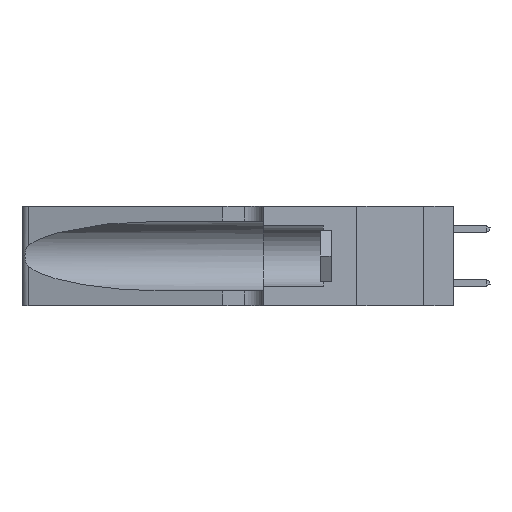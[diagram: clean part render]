
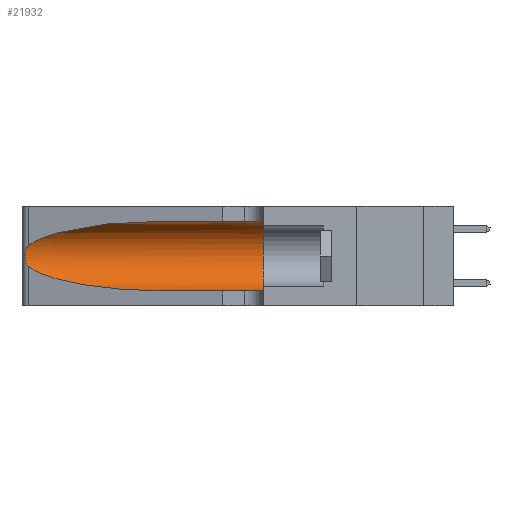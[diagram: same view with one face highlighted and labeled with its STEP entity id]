
A CAD part, left-side view. The second image highlights one B-rep face of the part: STEP entity #21932.
In plain terms, the highlighted cylindrical face has radius 3.308 mm (diameter 6.617 mm), a partial arc.
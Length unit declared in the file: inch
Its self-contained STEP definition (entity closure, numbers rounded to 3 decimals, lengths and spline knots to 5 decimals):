
#1064 = CARTESIAN_POINT ( 'NONE',  ( 0.25487, 1.22718, 0.22369 ) ) ;
#2345 = CARTESIAN_POINT ( 'NONE',  ( 0.25487, 1.22718, 0.22369 ) ) ;
#2739 = EDGE_CURVE ( 'NONE', #7046, #26798, #13587, .T. ) ;
#2786 = DIRECTION ( 'NONE',  ( 0., 0., -1. ) ) ;
#2940 = EDGE_CURVE ( 'NONE', #19266, #15660, #3195, .T. ) ;
#3195 = CIRCLE ( 'NONE', #27784, 0.13025 ) ;
#3874 = CARTESIAN_POINT ( 'NONE',  ( 0.25487, 1.22718, 0.22369 ) ) ;
#4031 = EDGE_CURVE ( 'NONE', #26867, #19266, #11959, .T. ) ;
#4232 = CYLINDRICAL_SURFACE ( 'NONE', #11273, 0.13025 ) ;
#5357 = CARTESIAN_POINT ( 'NONE',  ( 0.1305, 0.35, 0.31525 ) ) ;
#5538 = CARTESIAN_POINT ( 'NONE',  ( 0.26075, 1.23896, 0.178 ) ) ;
#5581 = VERTEX_POINT ( 'NONE', #11405 ) ;
#5630 = CARTESIAN_POINT ( 'NONE',  ( 0.26075, 1.23896, 0.19203 ) ) ;
#6467 = ORIENTED_EDGE ( 'NONE', *, *, #9641, .T. ) ;
#7046 = VERTEX_POINT ( 'NONE', #3874 ) ;
#7950 = CARTESIAN_POINT ( 'NONE',  ( 0.25854, 1.2359, 0.20912 ) ) ;
#8447 = CARTESIAN_POINT ( 'NONE',  ( 0.1305, 1.61858, 0.31525 ) ) ;
#8806 = EDGE_LOOP ( 'NONE', ( #25374, #16223, #6467, #10696, #26474, #26858 ) ) ;
#8916 = CARTESIAN_POINT ( 'NONE',  ( 0.25487, 1.22718, 0.14631 ) ) ;
#9152 = CARTESIAN_POINT ( 'NONE',  ( 0.1305, 0.35, 0.185 ) ) ;
#9641 = EDGE_CURVE ( 'NONE', #26798, #5581, #20882, .T. ) ;
#9998 = CARTESIAN_POINT ( 'NONE',  ( 0.25555, 1.22993, 0.14849 ) ) ;
#10171 = CARTESIAN_POINT ( 'NONE',  ( 0.25856, 1.23593, 0.16098 ) ) ;
#10696 = ORIENTED_EDGE ( 'NONE', *, *, #25628, .T. ) ;
#11273 = AXIS2_PLACEMENT_3D ( 'NONE', #22894, #16271, #2786 ) ;
#11405 = CARTESIAN_POINT ( 'NONE',  ( 0.1305, 0.72297, 0.05475 ) ) ;
#11941 = DIRECTION ( 'NONE',  ( 0., 0., 1. ) ) ;
#11959 = LINE ( 'NONE', #8447, #12990 ) ;
#12356 = LINE ( 'NONE', #23040, #23479 ) ;
#12990 = VECTOR ( 'NONE', #28362, 39.37008 ) ;
#13587 = B_SPLINE_CURVE_WITH_KNOTS ( 'NONE', 3,
 ( #1064, #21145, #18817, #21245, #7950, #23492, #5630, #5538, #25522, #10171, #21051, #23292, #9998, #16866 ),
 .UNSPECIFIED., .F., .F.,
 ( 4, 2, 2, 2, 2, 2, 4 ),
 ( 0., 0.00027, 0.00053, 0.00107, 0.0016, 0.00187, 0.00214 ),
 .UNSPECIFIED. ) ;
#15028 = CARTESIAN_POINT ( 'NONE',  ( 0.2373, 1.15595, 0.08982 ) ) ;
#15220 = CARTESIAN_POINT ( 'NONE',  ( 0.18966, 0.96281, 0.05475 ) ) ;
#15327 = CARTESIAN_POINT ( 'NONE',  ( 0.1305, 0.72297, 0.05475 ) ) ;
#15660 = VERTEX_POINT ( 'NONE', #19179 ) ;
#15718 = CARTESIAN_POINT ( 'NONE',  ( 0.2373, 1.15595, 0.28018 ) ) ;
#16223 = ORIENTED_EDGE ( 'NONE', *, *, #2739, .T. ) ;
#16271 = DIRECTION ( 'NONE',  ( 0., -1., 0. ) ) ;
#16866 = CARTESIAN_POINT ( 'NONE',  ( 0.25487, 1.22718, 0.14631 ) ) ;
#17584 = CARTESIAN_POINT ( 'NONE',  ( 0.1305, 0.72297, 0.31525 ) ) ;
#18536 = EDGE_CURVE ( 'NONE', #26867, #7046, #23041, .T. ) ;
#18817 = CARTESIAN_POINT ( 'NONE',  ( 0.25639, 1.23184, 0.21858 ) ) ;
#19179 = CARTESIAN_POINT ( 'NONE',  ( 0.1305, 0.35, 0.05475 ) ) ;
#19266 = VERTEX_POINT ( 'NONE', #5357 ) ;
#20882 =( BOUNDED_CURVE ( )  B_SPLINE_CURVE ( 3, ( #24077, #15028, #15220, #15327 ),
 .UNSPECIFIED., .F., .F. ) 
 B_SPLINE_CURVE_WITH_KNOTS ( ( 4, 4 ),
 ( 3.44316, 4.71239 ),
 .UNSPECIFIED. ) 
 CURVE ( )  GEOMETRIC_REPRESENTATION_ITEM ( )  RATIONAL_B_SPLINE_CURVE ( ( 1., 0.87, 0.87, 1. ) ) 
 REPRESENTATION_ITEM ( '' )  );
#21051 = CARTESIAN_POINT ( 'NONE',  ( 0.25789, 1.23486, 0.15765 ) ) ;
#21145 = CARTESIAN_POINT ( 'NONE',  ( 0.25555, 1.22994, 0.2215 ) ) ;
#21245 = CARTESIAN_POINT ( 'NONE',  ( 0.25787, 1.23484, 0.2124 ) ) ;
#21932 = ADVANCED_FACE ( 'NONE', ( #27868 ), #4232, .F. ) ;
#22651 = DIRECTION ( 'NONE',  ( 0., -1., 0. ) ) ;
#22728 = DIRECTION ( 'NONE',  ( 0., 1., 0. ) ) ;
#22894 = CARTESIAN_POINT ( 'NONE',  ( 0.1305, 1.61858, 0.185 ) ) ;
#23040 = CARTESIAN_POINT ( 'NONE',  ( 0.1305, 1.61858, 0.05475 ) ) ;
#23041 =( BOUNDED_CURVE ( )  B_SPLINE_CURVE ( 3, ( #17584, #28489, #15718, #2345 ),
 .UNSPECIFIED., .F., .F. ) 
 B_SPLINE_CURVE_WITH_KNOTS ( ( 4, 4 ),
 ( 1.5708, 2.84003 ),
 .UNSPECIFIED. ) 
 CURVE ( )  GEOMETRIC_REPRESENTATION_ITEM ( )  RATIONAL_B_SPLINE_CURVE ( ( 1., 0.87, 0.87, 1. ) ) 
 REPRESENTATION_ITEM ( '' )  );
#23292 = CARTESIAN_POINT ( 'NONE',  ( 0.25639, 1.23186, 0.15144 ) ) ;
#23479 = VECTOR ( 'NONE', #22651, 39.37008 ) ;
#23492 = CARTESIAN_POINT ( 'NONE',  ( 0.26018, 1.23835, 0.19895 ) ) ;
#24077 = CARTESIAN_POINT ( 'NONE',  ( 0.25487, 1.22718, 0.14631 ) ) ;
#25374 = ORIENTED_EDGE ( 'NONE', *, *, #18536, .T. ) ;
#25522 = CARTESIAN_POINT ( 'NONE',  ( 0.26017, 1.23833, 0.17102 ) ) ;
#25628 = EDGE_CURVE ( 'NONE', #5581, #15660, #12356, .T. ) ;
#26474 = ORIENTED_EDGE ( 'NONE', *, *, #2940, .F. ) ;
#26798 = VERTEX_POINT ( 'NONE', #8916 ) ;
#26858 = ORIENTED_EDGE ( 'NONE', *, *, #4031, .F. ) ;
#26863 = CARTESIAN_POINT ( 'NONE',  ( 0.1305, 0.72297, 0.31525 ) ) ;
#26867 = VERTEX_POINT ( 'NONE', #26863 ) ;
#27784 = AXIS2_PLACEMENT_3D ( 'NONE', #9152, #22728, #11941 ) ;
#27868 = FACE_OUTER_BOUND ( 'NONE', #8806, .T. ) ;
#28362 = DIRECTION ( 'NONE',  ( 0., -1., 0. ) ) ;
#28489 = CARTESIAN_POINT ( 'NONE',  ( 0.18966, 0.96281, 0.31525 ) ) ;
